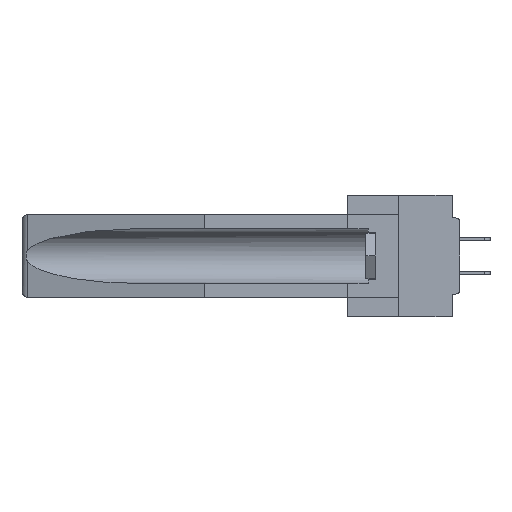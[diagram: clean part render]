
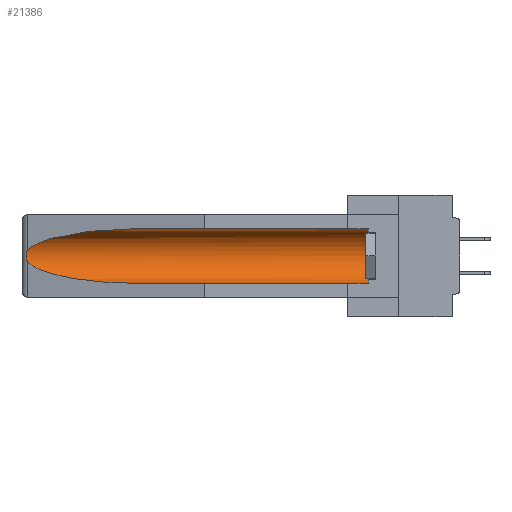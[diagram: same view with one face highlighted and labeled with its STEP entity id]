
A CAD part, left-side view. The second image highlights one B-rep face of the part: STEP entity #21386.
In plain terms, the highlighted cylindrical face has radius 2.857 mm (diameter 5.715 mm), a partial arc.
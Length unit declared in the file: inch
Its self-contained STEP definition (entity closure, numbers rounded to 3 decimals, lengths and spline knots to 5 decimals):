
#292 = CARTESIAN_POINT ( 'NONE',  ( 0.26537, 1.52718, -0.19328 ) ) ;
#341 = CYLINDRICAL_SURFACE ( 'NONE', #5282, 0.1125 ) ;
#620 = CARTESIAN_POINT ( 'NONE',  ( 0.26537, 1.52718, -0.14972 ) ) ;
#636 = B_SPLINE_CURVE_WITH_KNOTS ( 'NONE', 3,
 ( #1828, #4531, #26463, #10219, #18460, #23593, #26112, #12538, #17995, #20704 ),
 .UNSPECIFIED., .F., .F.,
 ( 4, 2, 2, 2, 4 ),
 ( 0., 0.00029, 0.00058, 0.00087, 0.00117 ),
 .UNSPECIFIED. ) ;
#1086 = VERTEX_POINT ( 'NONE', #32947 ) ;
#1828 = CARTESIAN_POINT ( 'NONE',  ( 0.26537, 1.52718, -0.14972 ) ) ;
#1834 = EDGE_CURVE ( 'NONE', #21882, #6032, #27706, .T. ) ;
#2245 = CARTESIAN_POINT ( 'NONE',  ( 0.25451, 1.48313, -0.09465 ) ) ;
#2729 = ORIENTED_EDGE ( 'NONE', *, *, #9310, .T. ) ;
#3166 = DIRECTION ( 'NONE',  ( 0., 1., 0. ) ) ;
#3588 = ORIENTED_EDGE ( 'NONE', *, *, #24496, .T. ) ;
#3867 = AXIS2_PLACEMENT_3D ( 'NONE', #12001, #28475, #17595 ) ;
#4531 = CARTESIAN_POINT ( 'NONE',  ( 0.26597, 1.52961, -0.15275 ) ) ;
#5282 = AXIS2_PLACEMENT_3D ( 'NONE', #26422, #18415, #10070 ) ;
#6032 = VERTEX_POINT ( 'NONE', #15409 ) ;
#6377 = EDGE_CURVE ( 'NONE', #34218, #21882, #636, .T. ) ;
#6659 = VERTEX_POINT ( 'NONE', #15971 ) ;
#6705 = ORIENTED_EDGE ( 'NONE', *, *, #1834, .T. ) ;
#7582 = CARTESIAN_POINT ( 'NONE',  ( 0.21114, 1.30732, -0.059 ) ) ;
#9075 = CARTESIAN_POINT ( 'NONE',  ( 0.26537, 1.52718, -0.19328 ) ) ;
#9252 = FACE_OUTER_BOUND ( 'NONE', #22049, .T. ) ;
#9306 = CARTESIAN_POINT ( 'NONE',  ( 0.155, 1.07973, -0.284 ) ) ;
#9310 = EDGE_CURVE ( 'NONE', #13951, #6659, #30112, .T. ) ;
#10070 = DIRECTION ( 'NONE',  ( 0., 0., 1. ) ) ;
#10219 = CARTESIAN_POINT ( 'NONE',  ( 0.2673, 1.5327, -0.16383 ) ) ;
#11242 = EDGE_CURVE ( 'NONE', #13951, #6032, #23139, .T. ) ;
#11929 = ORIENTED_EDGE ( 'NONE', *, *, #11242, .F. ) ;
#12001 = CARTESIAN_POINT ( 'NONE',  ( 0.155, 0.126, -0.1715 ) ) ;
#12213 = EDGE_CURVE ( 'NONE', #1086, #34218, #15420, .T. ) ;
#12538 = CARTESIAN_POINT ( 'NONE',  ( 0.26655, 1.53094, -0.18657 ) ) ;
#13588 = CARTESIAN_POINT ( 'NONE',  ( 0.155, 0.126, -0.284 ) ) ;
#13951 = VERTEX_POINT ( 'NONE', #13588 ) ;
#15282 = ORIENTED_EDGE ( 'NONE', *, *, #6377, .T. ) ;
#15409 = CARTESIAN_POINT ( 'NONE',  ( 0.155, 1.07973, -0.284 ) ) ;
#15420 =( BOUNDED_CURVE ( )  B_SPLINE_CURVE ( 3, ( #18207, #7582, #2245, #15676 ),
 .UNSPECIFIED., .F., .F. ) 
 B_SPLINE_CURVE_WITH_KNOTS ( ( 4, 4 ),
 ( 4.71239, 6.08839 ),
 .UNSPECIFIED. ) 
 CURVE ( )  GEOMETRIC_REPRESENTATION_ITEM ( )  RATIONAL_B_SPLINE_CURVE ( ( 1., 0.848, 0.848, 1. ) ) 
 REPRESENTATION_ITEM ( '' )  );
#15676 = CARTESIAN_POINT ( 'NONE',  ( 0.26537, 1.52718, -0.14972 ) ) ;
#15971 = CARTESIAN_POINT ( 'NONE',  ( 0.155, 0.126, -0.059 ) ) ;
#17192 = CARTESIAN_POINT ( 'NONE',  ( 0.21114, 1.30732, -0.284 ) ) ;
#17595 = DIRECTION ( 'NONE',  ( 0., 0., 1. ) ) ;
#17995 = CARTESIAN_POINT ( 'NONE',  ( 0.26597, 1.5296, -0.19026 ) ) ;
#18011 = VECTOR ( 'NONE', #3166, 39.37008 ) ;
#18207 = CARTESIAN_POINT ( 'NONE',  ( 0.155, 1.07973, -0.059 ) ) ;
#18415 = DIRECTION ( 'NONE',  ( 0., 1., 0. ) ) ;
#18460 = CARTESIAN_POINT ( 'NONE',  ( 0.2675, 1.53308, -0.16763 ) ) ;
#20704 = CARTESIAN_POINT ( 'NONE',  ( 0.26537, 1.52718, -0.19328 ) ) ;
#20908 = CARTESIAN_POINT ( 'NONE',  ( 0.155, -0.30754, -0.059 ) ) ;
#21386 = ADVANCED_FACE ( 'NONE', ( #9252 ), #341, .F. ) ;
#21882 = VERTEX_POINT ( 'NONE', #292 ) ;
#22049 = EDGE_LOOP ( 'NONE', ( #25710, #15282, #6705, #11929, #2729, #3588 ) ) ;
#22778 = CARTESIAN_POINT ( 'NONE',  ( 0.25451, 1.48313, -0.24835 ) ) ;
#23139 = LINE ( 'NONE', #29978, #18011 ) ;
#23593 = CARTESIAN_POINT ( 'NONE',  ( 0.2675, 1.53308, -0.17534 ) ) ;
#24496 = EDGE_CURVE ( 'NONE', #6659, #1086, #28062, .T. ) ;
#25710 = ORIENTED_EDGE ( 'NONE', *, *, #12213, .T. ) ;
#26112 = CARTESIAN_POINT ( 'NONE',  ( 0.2673, 1.53269, -0.17917 ) ) ;
#26422 = CARTESIAN_POINT ( 'NONE',  ( 0.155, -0.30754, -0.1715 ) ) ;
#26463 = CARTESIAN_POINT ( 'NONE',  ( 0.26654, 1.53092, -0.15636 ) ) ;
#27706 =( BOUNDED_CURVE ( )  B_SPLINE_CURVE ( 3, ( #9075, #22778, #17192, #9306 ),
 .UNSPECIFIED., .F., .F. ) 
 B_SPLINE_CURVE_WITH_KNOTS ( ( 4, 4 ),
 ( 0.1948, 1.5708 ),
 .UNSPECIFIED. ) 
 CURVE ( )  GEOMETRIC_REPRESENTATION_ITEM ( )  RATIONAL_B_SPLINE_CURVE ( ( 1., 0.848, 0.848, 1. ) ) 
 REPRESENTATION_ITEM ( '' )  );
#28062 = LINE ( 'NONE', #20908, #30162 ) ;
#28475 = DIRECTION ( 'NONE',  ( 0., -1., 0. ) ) ;
#29978 = CARTESIAN_POINT ( 'NONE',  ( 0.155, -0.30754, -0.284 ) ) ;
#30112 = CIRCLE ( 'NONE', #3867, 0.1125 ) ;
#30162 = VECTOR ( 'NONE', #31931, 39.37008 ) ;
#31931 = DIRECTION ( 'NONE',  ( 0., 1., 0. ) ) ;
#32947 = CARTESIAN_POINT ( 'NONE',  ( 0.155, 1.07973, -0.059 ) ) ;
#34218 = VERTEX_POINT ( 'NONE', #620 ) ;
